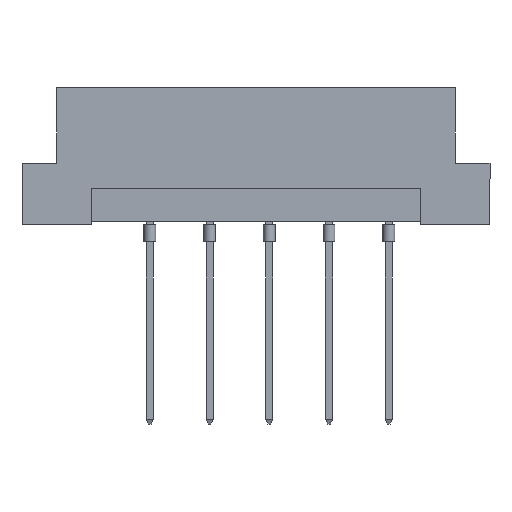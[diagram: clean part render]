
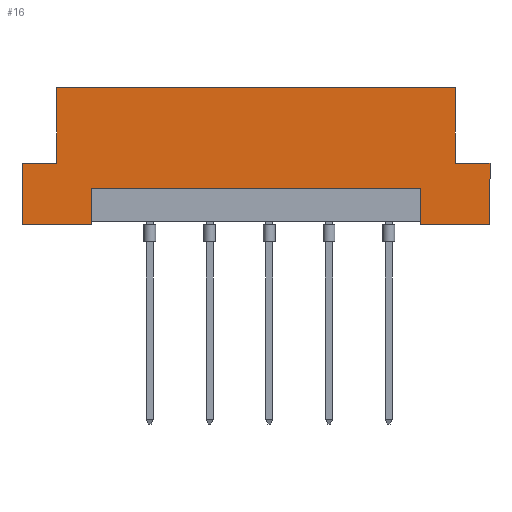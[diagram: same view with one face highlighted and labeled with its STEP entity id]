
A CAD part, front view. The second image highlights one B-rep face of the part: STEP entity #16.
In plain terms, the highlighted planar face has unit normal (0, -1, 0).
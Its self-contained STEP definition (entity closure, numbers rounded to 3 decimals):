
#16 = ADVANCED_FACE ( 'NONE', ( #62 ), #1358, .F. ) ;
#62 = FACE_OUTER_BOUND ( 'NONE', #420, .T. ) ;
#172 = LINE ( 'NONE', #4716, #995 ) ;
#309 = CARTESIAN_POINT ( 'NONE',  ( 19.9, -4.3, 0. ) ) ;
#346 = CARTESIAN_POINT ( 'NONE',  ( -19.9, -4.3, 11.6 ) ) ;
#420 = EDGE_LOOP ( 'NONE', ( #3757, #2391, #3161, #1044, #857, #2920, #1151, #1516, #1715, #4554, #2646, #2775 ) ) ;
#491 = CARTESIAN_POINT ( 'NONE',  ( 19.9, -4.3, 11.6 ) ) ;
#508 = EDGE_CURVE ( 'NONE', #4652, #4346, #5018, .T. ) ;
#523 = CARTESIAN_POINT ( 'NONE',  ( 19.9, -4.3, 11.6 ) ) ;
#526 = LINE ( 'NONE', #2509, #1920 ) ;
#532 = EDGE_CURVE ( 'NONE', #2022, #2565, #172, .T. ) ;
#536 = VERTEX_POINT ( 'NONE', #1824 ) ;
#550 = DIRECTION ( 'NONE',  ( 0., 0., 1. ) ) ;
#647 = LINE ( 'NONE', #3163, #3167 ) ;
#778 = CARTESIAN_POINT ( 'NONE',  ( -16.94, -4.3, 5.2 ) ) ;
#857 = ORIENTED_EDGE ( 'NONE', *, *, #3844, .F. ) ;
#902 = CARTESIAN_POINT ( 'NONE',  ( -14., -4.3, 3. ) ) ;
#923 = VERTEX_POINT ( 'NONE', #2499 ) ;
#995 = VECTOR ( 'NONE', #550, 1000. ) ;
#1044 = ORIENTED_EDGE ( 'NONE', *, *, #4547, .F. ) ;
#1151 = ORIENTED_EDGE ( 'NONE', *, *, #4179, .F. ) ;
#1221 = VERTEX_POINT ( 'NONE', #1569 ) ;
#1272 = VECTOR ( 'NONE', #3372, 1000. ) ;
#1285 = DIRECTION ( 'NONE',  ( 1., 0., 0. ) ) ;
#1296 = EDGE_CURVE ( 'NONE', #3383, #4645, #4872, .T. ) ;
#1358 = PLANE ( 'NONE',  #4811 ) ;
#1367 = LINE ( 'NONE', #523, #1272 ) ;
#1418 = DIRECTION ( 'NONE',  ( 0., 0., -1. ) ) ;
#1481 = DIRECTION ( 'NONE',  ( 1., 0., 0. ) ) ;
#1494 = DIRECTION ( 'NONE',  ( 0., 0., -1. ) ) ;
#1516 = ORIENTED_EDGE ( 'NONE', *, *, #5272, .F. ) ;
#1569 = CARTESIAN_POINT ( 'NONE',  ( -16.94, -4.3, 11.6 ) ) ;
#1694 = CARTESIAN_POINT ( 'NONE',  ( 19.9, -4.3, 0. ) ) ;
#1715 = ORIENTED_EDGE ( 'NONE', *, *, #2428, .F. ) ;
#1774 = VECTOR ( 'NONE', #5215, 1000. ) ;
#1824 = CARTESIAN_POINT ( 'NONE',  ( 14., -4.3, 0. ) ) ;
#1859 = VECTOR ( 'NONE', #1285, 1000. ) ;
#1884 = VECTOR ( 'NONE', #1997, 1000. ) ;
#1920 = VECTOR ( 'NONE', #3374, 1000. ) ;
#1953 = CARTESIAN_POINT ( 'NONE',  ( -19.9, -4.3, 5.2 ) ) ;
#1997 = DIRECTION ( 'NONE',  ( 0., 0., 1. ) ) ;
#2000 = VECTOR ( 'NONE', #1481, 1000. ) ;
#2022 = VERTEX_POINT ( 'NONE', #5267 ) ;
#2053 = LINE ( 'NONE', #778, #1884 ) ;
#2163 = CARTESIAN_POINT ( 'NONE',  ( 19.9, -4.3, 11.6 ) ) ;
#2183 = LINE ( 'NONE', #4212, #3298 ) ;
#2285 = EDGE_CURVE ( 'NONE', #536, #4957, #526, .T. ) ;
#2291 = EDGE_CURVE ( 'NONE', #4652, #4957, #2183, .T. ) ;
#2391 = ORIENTED_EDGE ( 'NONE', *, *, #2285, .F. ) ;
#2428 = EDGE_CURVE ( 'NONE', #3383, #4223, #4667, .T. ) ;
#2499 = CARTESIAN_POINT ( 'NONE',  ( 19.9, -4.3, 5.2 ) ) ;
#2509 = CARTESIAN_POINT ( 'NONE',  ( 14., -4.3, 0.2 ) ) ;
#2565 = VERTEX_POINT ( 'NONE', #5286 ) ;
#2594 = VERTEX_POINT ( 'NONE', #309 ) ;
#2613 = CARTESIAN_POINT ( 'NONE',  ( -19.9, -4.3, 0. ) ) ;
#2637 = DIRECTION ( 'NONE',  ( -1., 0., 0. ) ) ;
#2646 = ORIENTED_EDGE ( 'NONE', *, *, #4358, .T. ) ;
#2775 = ORIENTED_EDGE ( 'NONE', *, *, #508, .F. ) ;
#2787 = EDGE_CURVE ( 'NONE', #536, #2594, #4558, .T. ) ;
#2805 = CARTESIAN_POINT ( 'NONE',  ( 14., -4.3, 3. ) ) ;
#2920 = ORIENTED_EDGE ( 'NONE', *, *, #532, .T. ) ;
#3042 = CARTESIAN_POINT ( 'NONE',  ( -14., -4.3, 0.2 ) ) ;
#3161 = ORIENTED_EDGE ( 'NONE', *, *, #2787, .T. ) ;
#3163 = CARTESIAN_POINT ( 'NONE',  ( 19.9, -4.3, 5.2 ) ) ;
#3167 = VECTOR ( 'NONE', #3497, 1000. ) ;
#3298 = VECTOR ( 'NONE', #4997, 1000. ) ;
#3372 = DIRECTION ( 'NONE',  ( 0., 0., -1. ) ) ;
#3374 = DIRECTION ( 'NONE',  ( 0., 0., 1. ) ) ;
#3383 = VERTEX_POINT ( 'NONE', #1953 ) ;
#3497 = DIRECTION ( 'NONE',  ( 1., 0., 0. ) ) ;
#3545 = CARTESIAN_POINT ( 'NONE',  ( -14., -4.3, 0. ) ) ;
#3597 = LINE ( 'NONE', #5241, #1774 ) ;
#3678 = VECTOR ( 'NONE', #1418, 1000. ) ;
#3757 = ORIENTED_EDGE ( 'NONE', *, *, #2291, .T. ) ;
#3844 = EDGE_CURVE ( 'NONE', #2022, #923, #647, .T. ) ;
#3856 = CARTESIAN_POINT ( 'NONE',  ( -16.94, -4.3, 5.2 ) ) ;
#4179 = EDGE_CURVE ( 'NONE', #1221, #2565, #4697, .T. ) ;
#4212 = CARTESIAN_POINT ( 'NONE',  ( -14., -4.3, 3. ) ) ;
#4223 = VERTEX_POINT ( 'NONE', #3856 ) ;
#4277 = DIRECTION ( 'NONE',  ( 0., 1., 0. ) ) ;
#4345 = CARTESIAN_POINT ( 'NONE',  ( -19.9, -4.3, 5.2 ) ) ;
#4346 = VERTEX_POINT ( 'NONE', #3545 ) ;
#4358 = EDGE_CURVE ( 'NONE', #4645, #4346, #3597, .T. ) ;
#4430 = VECTOR ( 'NONE', #1494, 1000. ) ;
#4433 = VECTOR ( 'NONE', #4990, 1000. ) ;
#4547 = EDGE_CURVE ( 'NONE', #923, #2594, #1367, .T. ) ;
#4554 = ORIENTED_EDGE ( 'NONE', *, *, #1296, .T. ) ;
#4558 = LINE ( 'NONE', #1694, #4433 ) ;
#4645 = VERTEX_POINT ( 'NONE', #2613 ) ;
#4652 = VERTEX_POINT ( 'NONE', #902 ) ;
#4667 = LINE ( 'NONE', #4345, #2000 ) ;
#4697 = LINE ( 'NONE', #2163, #1859 ) ;
#4716 = CARTESIAN_POINT ( 'NONE',  ( 16.94, -4.3, 5.2 ) ) ;
#4811 = AXIS2_PLACEMENT_3D ( 'NONE', #491, #4277, #2637 ) ;
#4872 = LINE ( 'NONE', #346, #4430 ) ;
#4957 = VERTEX_POINT ( 'NONE', #2805 ) ;
#4990 = DIRECTION ( 'NONE',  ( 1., 0., 0. ) ) ;
#4997 = DIRECTION ( 'NONE',  ( 1., 0., 0. ) ) ;
#5018 = LINE ( 'NONE', #3042, #3678 ) ;
#5215 = DIRECTION ( 'NONE',  ( 1., 0., 0. ) ) ;
#5241 = CARTESIAN_POINT ( 'NONE',  ( 19.9, -4.3, 0. ) ) ;
#5267 = CARTESIAN_POINT ( 'NONE',  ( 16.94, -4.3, 5.2 ) ) ;
#5272 = EDGE_CURVE ( 'NONE', #4223, #1221, #2053, .T. ) ;
#5286 = CARTESIAN_POINT ( 'NONE',  ( 16.94, -4.3, 11.6 ) ) ;
